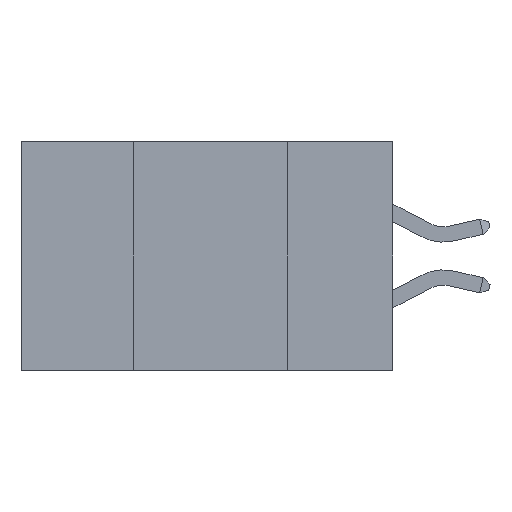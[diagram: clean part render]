
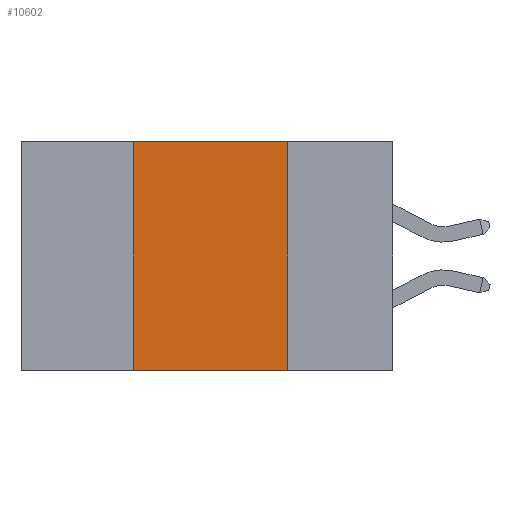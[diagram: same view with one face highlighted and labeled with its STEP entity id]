
A CAD part, left-side view. The second image highlights one B-rep face of the part: STEP entity #10602.
In plain terms, the highlighted planar face has unit normal (-1, 0, 0).
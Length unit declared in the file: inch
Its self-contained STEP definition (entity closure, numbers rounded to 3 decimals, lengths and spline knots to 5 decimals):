
#1324 = PLANE ( 'NONE',  #18465 ) ;
#1389 = CARTESIAN_POINT ( 'NONE',  ( 0., 0.6, 0. ) ) ;
#1636 = CARTESIAN_POINT ( 'NONE',  ( 0., 0.17, 0. ) ) ;
#1711 = VECTOR ( 'NONE', #2340, 39.37008 ) ;
#1975 = CARTESIAN_POINT ( 'NONE',  ( 0., 0.17, 0. ) ) ;
#2277 = LINE ( 'NONE', #17739, #1711 ) ;
#2340 = DIRECTION ( 'NONE',  ( 0., -1., 0. ) ) ;
#3141 = DIRECTION ( 'NONE',  ( 0., 0., -1. ) ) ;
#3394 = DIRECTION ( 'NONE',  ( 0., 0., -1. ) ) ;
#4197 = EDGE_CURVE ( 'NONE', #4926, #11245, #11127, .T. ) ;
#4793 = ORIENTED_EDGE ( 'NONE', *, *, #4197, .F. ) ;
#4926 = VERTEX_POINT ( 'NONE', #13473 ) ;
#5580 = VERTEX_POINT ( 'NONE', #1975 ) ;
#6722 = VECTOR ( 'NONE', #3394, 39.37008 ) ;
#7070 = VECTOR ( 'NONE', #12626, 39.37008 ) ;
#7257 = LINE ( 'NONE', #1636, #6722 ) ;
#7260 = EDGE_LOOP ( 'NONE', ( #17950, #10097, #4793, #17526 ) ) ;
#7710 = EDGE_CURVE ( 'NONE', #5580, #10685, #7257, .T. ) ;
#8637 = CARTESIAN_POINT ( 'NONE',  ( 0., 0.17, -0.37 ) ) ;
#9844 = EDGE_CURVE ( 'NONE', #11245, #5580, #2277, .T. ) ;
#10097 = ORIENTED_EDGE ( 'NONE', *, *, #9844, .F. ) ;
#10602 = ADVANCED_FACE ( 'NONE', ( #17012 ), #1324, .F. ) ;
#10685 = VERTEX_POINT ( 'NONE', #8637 ) ;
#11127 = LINE ( 'NONE', #18768, #7070 ) ;
#11245 = VERTEX_POINT ( 'NONE', #15163 ) ;
#12005 = LINE ( 'NONE', #14547, #19916 ) ;
#12626 = DIRECTION ( 'NONE',  ( 0., 0., 1. ) ) ;
#12908 = DIRECTION ( 'NONE',  ( 0., -1., 0. ) ) ;
#13473 = CARTESIAN_POINT ( 'NONE',  ( 0., 0.42, -0.37 ) ) ;
#13508 = DIRECTION ( 'NONE',  ( 1., 0., 0. ) ) ;
#14547 = CARTESIAN_POINT ( 'NONE',  ( 0., 0.6, -0.37 ) ) ;
#15163 = CARTESIAN_POINT ( 'NONE',  ( 0., 0.42, 0. ) ) ;
#17012 = FACE_OUTER_BOUND ( 'NONE', #7260, .T. ) ;
#17526 = ORIENTED_EDGE ( 'NONE', *, *, #18424, .T. ) ;
#17739 = CARTESIAN_POINT ( 'NONE',  ( 0., 0.6, 0. ) ) ;
#17950 = ORIENTED_EDGE ( 'NONE', *, *, #7710, .F. ) ;
#18424 = EDGE_CURVE ( 'NONE', #4926, #10685, #12005, .T. ) ;
#18465 = AXIS2_PLACEMENT_3D ( 'NONE', #1389, #13508, #3141 ) ;
#18768 = CARTESIAN_POINT ( 'NONE',  ( 0., 0.42, 0. ) ) ;
#19916 = VECTOR ( 'NONE', #12908, 39.37008 ) ;
